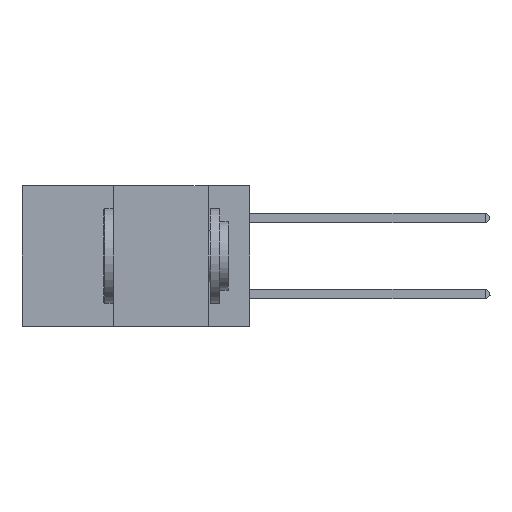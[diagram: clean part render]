
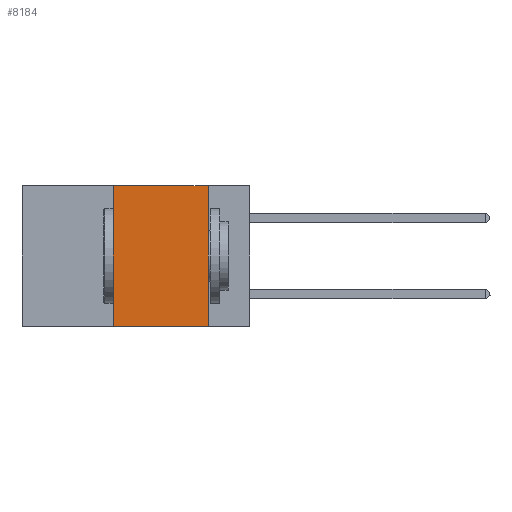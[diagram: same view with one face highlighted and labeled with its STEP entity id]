
A CAD part, left-side view. The second image highlights one B-rep face of the part: STEP entity #8184.
In plain terms, the highlighted planar face has unit normal (-1, 0, 0).
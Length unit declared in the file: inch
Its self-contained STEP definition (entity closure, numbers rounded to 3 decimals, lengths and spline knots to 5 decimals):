
#33 = EDGE_LOOP ( 'NONE', ( #12742, #17969, #2290, #293 ) ) ;
#121 = LINE ( 'NONE', #11224, #15697 ) ;
#293 = ORIENTED_EDGE ( 'NONE', *, *, #17601, .T. ) ;
#429 = FACE_OUTER_BOUND ( 'NONE', #33, .T. ) ;
#1142 = CARTESIAN_POINT ( 'NONE',  ( 0., 0.6, 0. ) ) ;
#1254 = VERTEX_POINT ( 'NONE', #14097 ) ;
#1321 = DIRECTION ( 'NONE',  ( 0., -1., 0. ) ) ;
#2290 = ORIENTED_EDGE ( 'NONE', *, *, #11521, .F. ) ;
#2726 = DIRECTION ( 'NONE',  ( 0., -1., 0. ) ) ;
#2802 = CARTESIAN_POINT ( 'NONE',  ( 0., 0.6, 0. ) ) ;
#4204 = VERTEX_POINT ( 'NONE', #18460 ) ;
#4900 = DIRECTION ( 'NONE',  ( 0., 0., 1. ) ) ;
#5534 = LINE ( 'NONE', #16348, #12573 ) ;
#6288 = AXIS2_PLACEMENT_3D ( 'NONE', #2802, #11939, #10116 ) ;
#7492 = VECTOR ( 'NONE', #4900, 39.37008 ) ;
#8184 = ADVANCED_FACE ( 'NONE', ( #429 ), #11627, .F. ) ;
#10116 = DIRECTION ( 'NONE',  ( 0., 0., -1. ) ) ;
#10635 = CARTESIAN_POINT ( 'NONE',  ( 0., 0.36, 0. ) ) ;
#10920 = CARTESIAN_POINT ( 'NONE',  ( 0., 0.36, -0.37 ) ) ;
#11081 = LINE ( 'NONE', #1142, #12693 ) ;
#11224 = CARTESIAN_POINT ( 'NONE',  ( 0., 0.11, 0. ) ) ;
#11244 = EDGE_CURVE ( 'NONE', #4204, #13701, #11081, .T. ) ;
#11521 = EDGE_CURVE ( 'NONE', #18915, #4204, #13143, .T. ) ;
#11627 = PLANE ( 'NONE',  #6288 ) ;
#11939 = DIRECTION ( 'NONE',  ( 1., 0., 0. ) ) ;
#12573 = VECTOR ( 'NONE', #1321, 39.37008 ) ;
#12579 = EDGE_CURVE ( 'NONE', #13701, #1254, #121, .T. ) ;
#12693 = VECTOR ( 'NONE', #2726, 39.37008 ) ;
#12742 = ORIENTED_EDGE ( 'NONE', *, *, #12579, .F. ) ;
#13143 = LINE ( 'NONE', #10635, #7492 ) ;
#13701 = VERTEX_POINT ( 'NONE', #17158 ) ;
#14097 = CARTESIAN_POINT ( 'NONE',  ( 0., 0.11, -0.37 ) ) ;
#15697 = VECTOR ( 'NONE', #16052, 39.37008 ) ;
#16052 = DIRECTION ( 'NONE',  ( 0., 0., -1. ) ) ;
#16348 = CARTESIAN_POINT ( 'NONE',  ( 0., 0.6, -0.37 ) ) ;
#17158 = CARTESIAN_POINT ( 'NONE',  ( 0., 0.11, 0. ) ) ;
#17601 = EDGE_CURVE ( 'NONE', #18915, #1254, #5534, .T. ) ;
#17969 = ORIENTED_EDGE ( 'NONE', *, *, #11244, .F. ) ;
#18460 = CARTESIAN_POINT ( 'NONE',  ( 0., 0.36, 0. ) ) ;
#18915 = VERTEX_POINT ( 'NONE', #10920 ) ;
